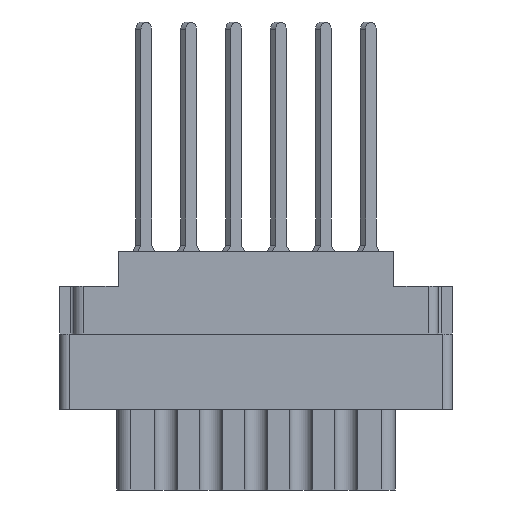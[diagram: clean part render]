
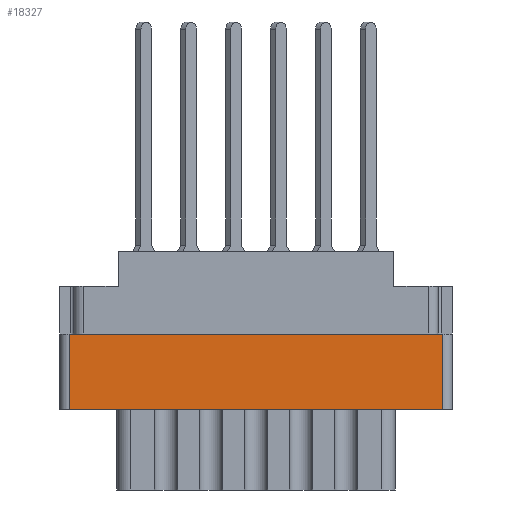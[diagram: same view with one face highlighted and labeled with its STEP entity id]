
A CAD part, front view. The second image highlights one B-rep face of the part: STEP entity #18327.
In plain terms, the highlighted planar face has unit normal (0, -1, 0).
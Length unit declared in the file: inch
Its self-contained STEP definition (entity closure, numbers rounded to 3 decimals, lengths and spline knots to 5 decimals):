
#843 = LINE ( 'NONE', #23039, #9539 ) ;
#905 = DIRECTION ( 'NONE',  ( 1., 0., 0. ) ) ;
#1593 = VERTEX_POINT ( 'NONE', #11724 ) ;
#3885 = EDGE_CURVE ( 'NONE', #1593, #20611, #13121, .T. ) ;
#3886 = DIRECTION ( 'NONE',  ( 0., -1., 0. ) ) ;
#4292 = AXIS2_PLACEMENT_3D ( 'NONE', #20246, #3886, #11158 ) ;
#4490 = CARTESIAN_POINT ( 'NONE',  ( -0.656, -0.343, -0.277 ) ) ;
#4601 = EDGE_CURVE ( 'NONE', #22697, #13591, #9966, .T. ) ;
#5680 = FACE_OUTER_BOUND ( 'NONE', #21849, .T. ) ;
#6191 = CARTESIAN_POINT ( 'NONE',  ( 0.624, -0.343, -0.277 ) ) ;
#6271 = VECTOR ( 'NONE', #16343, 39.37008 ) ;
#7423 = EDGE_CURVE ( 'NONE', #20611, #22697, #12759, .T. ) ;
#7567 = VECTOR ( 'NONE', #9537, 39.37008 ) ;
#9537 = DIRECTION ( 'NONE',  ( -1., 0., 0. ) ) ;
#9539 = VECTOR ( 'NONE', #12053, 39.37008 ) ;
#9966 = LINE ( 'NONE', #4490, #12926 ) ;
#11158 = DIRECTION ( 'NONE',  ( 0., 0., -1. ) ) ;
#11724 = CARTESIAN_POINT ( 'NONE',  ( 0.624, -0.343, -0.529 ) ) ;
#12053 = DIRECTION ( 'NONE',  ( 0., 0., 1. ) ) ;
#12059 = ORIENTED_EDGE ( 'NONE', *, *, #7423, .F. ) ;
#12759 = LINE ( 'NONE', #12999, #6271 ) ;
#12926 = VECTOR ( 'NONE', #905, 39.37008 ) ;
#12956 = PLANE ( 'NONE',  #4292 ) ;
#12999 = CARTESIAN_POINT ( 'NONE',  ( -0.624, -0.343, -0.798 ) ) ;
#13121 = LINE ( 'NONE', #22204, #7567 ) ;
#13591 = VERTEX_POINT ( 'NONE', #6191 ) ;
#16343 = DIRECTION ( 'NONE',  ( 0., 0., 1. ) ) ;
#17365 = ORIENTED_EDGE ( 'NONE', *, *, #3885, .F. ) ;
#18327 = ADVANCED_FACE ( 'NONE', ( #5680 ), #12956, .T. ) ;
#20246 = CARTESIAN_POINT ( 'NONE',  ( -0.624, -0.343, -0.798 ) ) ;
#20611 = VERTEX_POINT ( 'NONE', #22706 ) ;
#21059 = CARTESIAN_POINT ( 'NONE',  ( -0.624, -0.343, -0.277 ) ) ;
#21849 = EDGE_LOOP ( 'NONE', ( #12059, #17365, #23444, #22547 ) ) ;
#22204 = CARTESIAN_POINT ( 'NONE',  ( 0.624, -0.343, -0.529 ) ) ;
#22547 = ORIENTED_EDGE ( 'NONE', *, *, #4601, .F. ) ;
#22697 = VERTEX_POINT ( 'NONE', #21059 ) ;
#22706 = CARTESIAN_POINT ( 'NONE',  ( -0.624, -0.343, -0.529 ) ) ;
#22992 = EDGE_CURVE ( 'NONE', #1593, #13591, #843, .T. ) ;
#23039 = CARTESIAN_POINT ( 'NONE',  ( 0.624, -0.343, -0.798 ) ) ;
#23444 = ORIENTED_EDGE ( 'NONE', *, *, #22992, .T. ) ;
